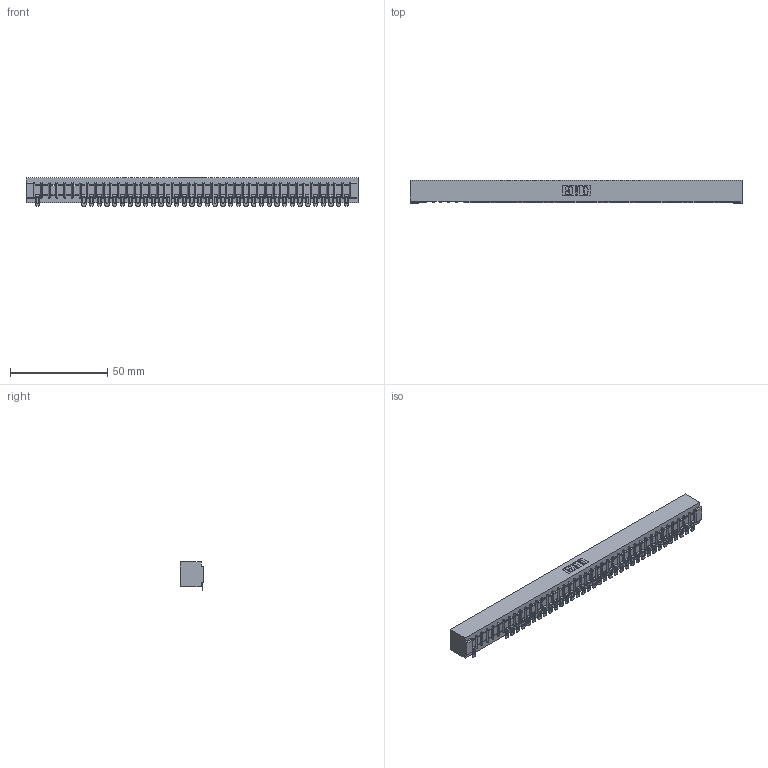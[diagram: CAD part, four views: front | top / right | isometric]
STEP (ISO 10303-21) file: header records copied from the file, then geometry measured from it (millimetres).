
FILE_DESCRIPTION (( 'STEP AP203' ), '1' );
FILE_NAME ('357-041-554-101.STEP', '2018-08-11T07:19:17', ( '' ), ( '' ), 'SwSTEP 2.0', 'SolidWorks 2016', '' );
FILE_SCHEMA (( 'CONFIG_CONTROL_DESIGN' ));
Length unit declared in the file: inch
Products named in the file (3): 307 Part_No Mounting Lugs; 307-290-002_554; 357-041-554-101
Assembly tree (37 placements, depth 2):
  357-041-554-101
    307 Part_No Mounting Lugs
    307-290-002_554  x36
Bounding box: 170.33 x 12.01 x 14.52 mm (x, y, z)
Volume: 18646.3 mm3; surface area: 22984.6 mm2
Topology: 37 solids, 37 shells, 3168 faces, 9727 edges, 6370 vertices
Faces by surface type: plane 1782, cylinder 1302, sphere 84
Entity records: 35799 total; most frequent: CARTESIAN_POINT 6061, ORIENTED_EDGE 6056, DIRECTION 5888, EDGE_CURVE 3028, VECTOR 2314, LINE 2314, VERTEX_POINT 1960, AXIS2_PLACEMENT_3D 1787
